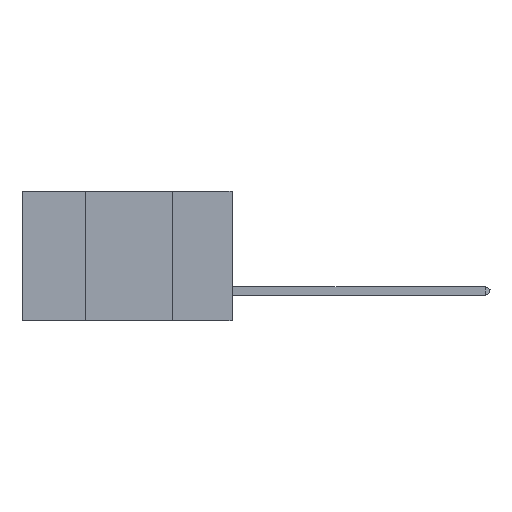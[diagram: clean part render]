
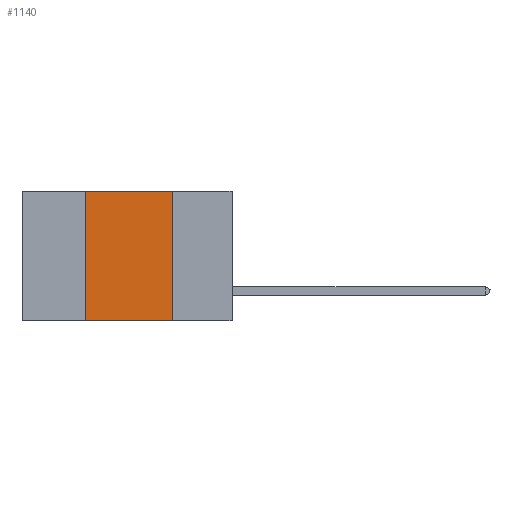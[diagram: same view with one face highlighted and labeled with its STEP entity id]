
A CAD part, left-side view. The second image highlights one B-rep face of the part: STEP entity #1140.
In plain terms, the highlighted planar face has unit normal (-1, 0, 0).
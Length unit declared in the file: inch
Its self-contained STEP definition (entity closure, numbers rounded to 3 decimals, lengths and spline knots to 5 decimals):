
#518 = EDGE_CURVE ( 'NONE', #835, #15500, #9032, .T. ) ;
#835 = VERTEX_POINT ( 'NONE', #12291 ) ;
#1140 = ADVANCED_FACE ( 'NONE', ( #23048 ), #23851, .F. ) ;
#1747 = LINE ( 'NONE', #4860, #29474 ) ;
#2320 = DIRECTION ( 'NONE',  ( 0., 0., -1. ) ) ;
#3811 = DIRECTION ( 'NONE',  ( 0., 0., 1. ) ) ;
#4860 = CARTESIAN_POINT ( 'NONE',  ( 0., 0.6, 0. ) ) ;
#5140 = EDGE_CURVE ( 'NONE', #6647, #15500, #14544, .T. ) ;
#6647 = VERTEX_POINT ( 'NONE', #19913 ) ;
#6874 = CARTESIAN_POINT ( 'NONE',  ( 0., 0.42, 0. ) ) ;
#7886 = VECTOR ( 'NONE', #3811, 39.37008 ) ;
#9032 = LINE ( 'NONE', #10439, #34476 ) ;
#10439 = CARTESIAN_POINT ( 'NONE',  ( 0., 0.6, -0.37 ) ) ;
#12043 = AXIS2_PLACEMENT_3D ( 'NONE', #26758, #19213, #22813 ) ;
#12291 = CARTESIAN_POINT ( 'NONE',  ( 0., 0.42, -0.37 ) ) ;
#12320 = VERTEX_POINT ( 'NONE', #27005 ) ;
#14544 = LINE ( 'NONE', #19971, #19505 ) ;
#14959 = EDGE_LOOP ( 'NONE', ( #36098, #31502, #30549, #32182 ) ) ;
#15500 = VERTEX_POINT ( 'NONE', #20972 ) ;
#19213 = DIRECTION ( 'NONE',  ( 1., 0., 0. ) ) ;
#19505 = VECTOR ( 'NONE', #2320, 39.37008 ) ;
#19913 = CARTESIAN_POINT ( 'NONE',  ( 0., 0.17, 0. ) ) ;
#19971 = CARTESIAN_POINT ( 'NONE',  ( 0., 0.17, 0. ) ) ;
#20972 = CARTESIAN_POINT ( 'NONE',  ( 0., 0.17, -0.37 ) ) ;
#22813 = DIRECTION ( 'NONE',  ( 0., 0., -1. ) ) ;
#23048 = FACE_OUTER_BOUND ( 'NONE', #14959, .T. ) ;
#23851 = PLANE ( 'NONE',  #12043 ) ;
#24180 = LINE ( 'NONE', #6874, #7886 ) ;
#26251 = EDGE_CURVE ( 'NONE', #12320, #6647, #1747, .T. ) ;
#26758 = CARTESIAN_POINT ( 'NONE',  ( 0., 0.6, 0. ) ) ;
#27005 = CARTESIAN_POINT ( 'NONE',  ( 0., 0.42, 0. ) ) ;
#29474 = VECTOR ( 'NONE', #33917, 39.37008 ) ;
#30549 = ORIENTED_EDGE ( 'NONE', *, *, #34326, .F. ) ;
#31502 = ORIENTED_EDGE ( 'NONE', *, *, #26251, .F. ) ;
#32182 = ORIENTED_EDGE ( 'NONE', *, *, #518, .T. ) ;
#33665 = DIRECTION ( 'NONE',  ( 0., -1., 0. ) ) ;
#33917 = DIRECTION ( 'NONE',  ( 0., -1., 0. ) ) ;
#34326 = EDGE_CURVE ( 'NONE', #835, #12320, #24180, .T. ) ;
#34476 = VECTOR ( 'NONE', #33665, 39.37008 ) ;
#36098 = ORIENTED_EDGE ( 'NONE', *, *, #5140, .F. ) ;
